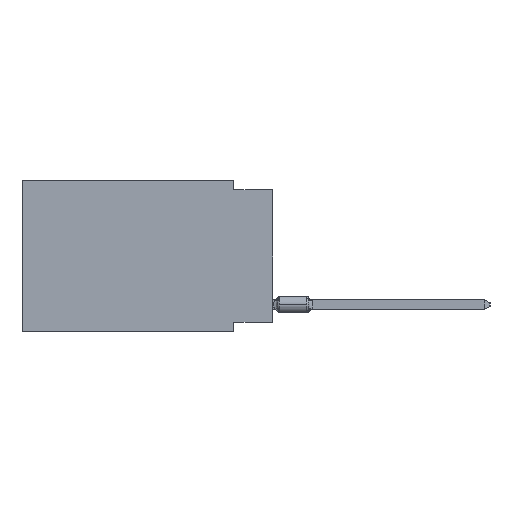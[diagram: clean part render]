
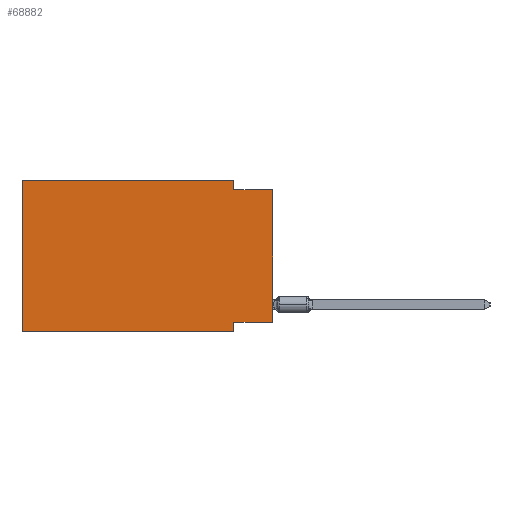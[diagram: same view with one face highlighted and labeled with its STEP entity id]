
A CAD part, left-side view. The second image highlights one B-rep face of the part: STEP entity #68882.
In plain terms, the highlighted planar face has unit normal (-1, 0, 0).
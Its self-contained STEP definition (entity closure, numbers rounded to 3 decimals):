
#550 = EDGE_CURVE ( 'NONE', #24494, #39222, #64120, .T. ) ;
#769 = LINE ( 'NONE', #38996, #74314 ) ;
#3881 = CARTESIAN_POINT ( 'NONE',  ( 0., 16.383, 0. ) ) ;
#4710 = AXIS2_PLACEMENT_3D ( 'NONE', #42528, #73752, #24014 ) ;
#4969 = LINE ( 'NONE', #28812, #20704 ) ;
#7028 = FACE_OUTER_BOUND ( 'NONE', #23731, .T. ) ;
#11243 = VECTOR ( 'NONE', #38233, 1000. ) ;
#13135 = LINE ( 'NONE', #32047, #11243 ) ;
#16074 = ORIENTED_EDGE ( 'NONE', *, *, #22622, .F. ) ;
#16927 = DIRECTION ( 'NONE',  ( 0., 0., -1. ) ) ;
#17300 = EDGE_CURVE ( 'NONE', #24494, #63704, #74574, .T. ) ;
#17599 = EDGE_CURVE ( 'NONE', #29761, #79820, #80937, .T. ) ;
#20159 = ORIENTED_EDGE ( 'NONE', *, *, #62431, .F. ) ;
#20161 = DIRECTION ( 'NONE',  ( 0., 0., 1. ) ) ;
#20347 = VECTOR ( 'NONE', #79128, 1000. ) ;
#20704 = VECTOR ( 'NONE', #30034, 1000. ) ;
#22334 = EDGE_CURVE ( 'NONE', #39222, #61732, #4969, .T. ) ;
#22622 = EDGE_CURVE ( 'NONE', #79820, #63704, #13135, .T. ) ;
#23510 = CARTESIAN_POINT ( 'NONE',  ( 0., 2.54, 0. ) ) ;
#23731 = EDGE_LOOP ( 'NONE', ( #51627, #47614, #20159, #53080, #62159, #33634, #16074, #66601 ) ) ;
#24014 = DIRECTION ( 'NONE',  ( 0., 0., -1. ) ) ;
#24494 = VERTEX_POINT ( 'NONE', #40049 ) ;
#25759 = CARTESIAN_POINT ( 'NONE',  ( 0., 0., -9.271 ) ) ;
#26730 = PLANE ( 'NONE',  #4710 ) ;
#28812 = CARTESIAN_POINT ( 'NONE',  ( 0., 16.383, 0. ) ) ;
#29761 = VERTEX_POINT ( 'NONE', #25759 ) ;
#30034 = DIRECTION ( 'NONE',  ( 0., -1., 0. ) ) ;
#32047 = CARTESIAN_POINT ( 'NONE',  ( 0., 2.54, -9.906 ) ) ;
#33634 = ORIENTED_EDGE ( 'NONE', *, *, #17300, .T. ) ;
#36605 = DIRECTION ( 'NONE',  ( 0., 1., 0. ) ) ;
#37397 = CARTESIAN_POINT ( 'NONE',  ( 0., 2.54, -9.271 ) ) ;
#37498 = VECTOR ( 'NONE', #36605, 1000. ) ;
#37801 = CARTESIAN_POINT ( 'NONE',  ( 0., 0., -9.271 ) ) ;
#38233 = DIRECTION ( 'NONE',  ( 0., 0., -1. ) ) ;
#38996 = CARTESIAN_POINT ( 'NONE',  ( 0., 0., -0.635 ) ) ;
#39222 = VERTEX_POINT ( 'NONE', #3881 ) ;
#40049 = CARTESIAN_POINT ( 'NONE',  ( 0., 16.383, -9.906 ) ) ;
#42528 = CARTESIAN_POINT ( 'NONE',  ( 0., 16.383, 0. ) ) ;
#45760 = VECTOR ( 'NONE', #59216, 1000. ) ;
#47271 = CARTESIAN_POINT ( 'NONE',  ( 0., 0., 0. ) ) ;
#47614 = ORIENTED_EDGE ( 'NONE', *, *, #64506, .F. ) ;
#47656 = CARTESIAN_POINT ( 'NONE',  ( 0., 2.54, 0. ) ) ;
#49370 = LINE ( 'NONE', #23510, #58366 ) ;
#51627 = ORIENTED_EDGE ( 'NONE', *, *, #54044, .T. ) ;
#52844 = DIRECTION ( 'NONE',  ( 0., -1., 0. ) ) ;
#53080 = ORIENTED_EDGE ( 'NONE', *, *, #22334, .F. ) ;
#54044 = EDGE_CURVE ( 'NONE', #29761, #70840, #76873, .T. ) ;
#54759 = CARTESIAN_POINT ( 'NONE',  ( 0., 0., -0.635 ) ) ;
#58366 = VECTOR ( 'NONE', #16927, 1000. ) ;
#59216 = DIRECTION ( 'NONE',  ( 0., 0., 1. ) ) ;
#59226 = CARTESIAN_POINT ( 'NONE',  ( 0., 2.54, -0.635 ) ) ;
#61732 = VERTEX_POINT ( 'NONE', #47656 ) ;
#61868 = CARTESIAN_POINT ( 'NONE',  ( 0., 16.383, -9.906 ) ) ;
#62159 = ORIENTED_EDGE ( 'NONE', *, *, #550, .F. ) ;
#62431 = EDGE_CURVE ( 'NONE', #61732, #64165, #49370, .T. ) ;
#63704 = VERTEX_POINT ( 'NONE', #77812 ) ;
#64120 = LINE ( 'NONE', #76054, #79361 ) ;
#64165 = VERTEX_POINT ( 'NONE', #59226 ) ;
#64506 = EDGE_CURVE ( 'NONE', #64165, #70840, #769, .T. ) ;
#66601 = ORIENTED_EDGE ( 'NONE', *, *, #17599, .F. ) ;
#68882 = ADVANCED_FACE ( 'NONE', ( #7028 ), #26730, .F. ) ;
#70840 = VERTEX_POINT ( 'NONE', #54759 ) ;
#73752 = DIRECTION ( 'NONE',  ( 1., 0., 0. ) ) ;
#74314 = VECTOR ( 'NONE', #52844, 1000. ) ;
#74574 = LINE ( 'NONE', #61868, #20347 ) ;
#76054 = CARTESIAN_POINT ( 'NONE',  ( 0., 16.383, 0. ) ) ;
#76873 = LINE ( 'NONE', #47271, #45760 ) ;
#77812 = CARTESIAN_POINT ( 'NONE',  ( 0., 2.54, -9.906 ) ) ;
#79128 = DIRECTION ( 'NONE',  ( 0., -1., 0. ) ) ;
#79361 = VECTOR ( 'NONE', #20161, 1000. ) ;
#79820 = VERTEX_POINT ( 'NONE', #37397 ) ;
#80937 = LINE ( 'NONE', #37801, #37498 ) ;
